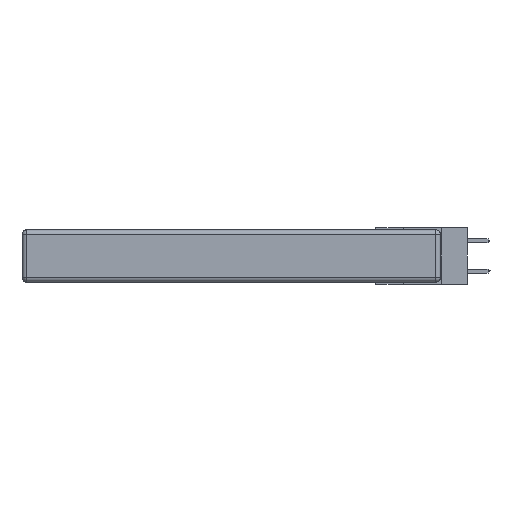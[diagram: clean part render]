
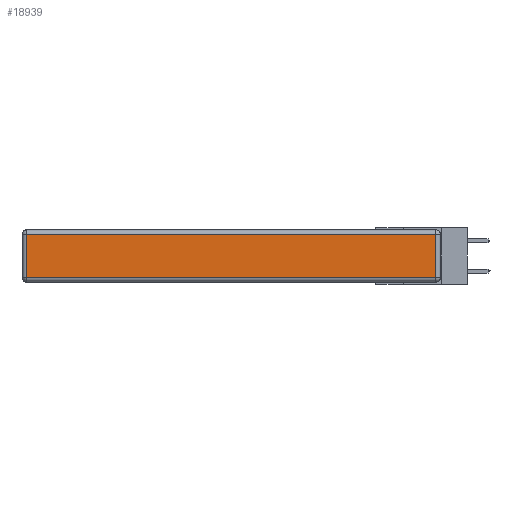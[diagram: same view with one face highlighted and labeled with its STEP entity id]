
A CAD part, left-side view. The second image highlights one B-rep face of the part: STEP entity #18939.
In plain terms, the highlighted planar face has unit normal (-1, 0, 0).
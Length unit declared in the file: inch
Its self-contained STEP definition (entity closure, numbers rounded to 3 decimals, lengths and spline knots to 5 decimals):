
#454 = ORIENTED_EDGE ( 'NONE', *, *, #20297, .T. ) ;
#1359 = ORIENTED_EDGE ( 'NONE', *, *, #7262, .T. ) ;
#4523 = AXIS2_PLACEMENT_3D ( 'NONE', #9905, #8316, #6566 ) ;
#4576 = CARTESIAN_POINT ( 'NONE',  ( 0., 2.72, -0.343 ) ) ;
#4876 = CARTESIAN_POINT ( 'NONE',  ( 0., 0.03, -0.313 ) ) ;
#4912 = FACE_OUTER_BOUND ( 'NONE', #19882, .T. ) ;
#5044 = CARTESIAN_POINT ( 'NONE',  ( 0., 0.03, -0.343 ) ) ;
#5182 = ORIENTED_EDGE ( 'NONE', *, *, #13146, .T. ) ;
#5830 = VECTOR ( 'NONE', #19994, 39.37008 ) ;
#6077 = DIRECTION ( 'NONE',  ( 0., 0., -1. ) ) ;
#6189 = CARTESIAN_POINT ( 'NONE',  ( 0., 0.03, -0.03 ) ) ;
#6566 = DIRECTION ( 'NONE',  ( 0., 0., 1. ) ) ;
#6700 = ORIENTED_EDGE ( 'NONE', *, *, #9604, .T. ) ;
#7262 = EDGE_CURVE ( 'NONE', #7684, #8375, #20512, .T. ) ;
#7684 = VERTEX_POINT ( 'NONE', #13353 ) ;
#8082 = VECTOR ( 'NONE', #8680, 39.37008 ) ;
#8316 = DIRECTION ( 'NONE',  ( -1., 0., 0. ) ) ;
#8375 = VERTEX_POINT ( 'NONE', #4876 ) ;
#8534 = LINE ( 'NONE', #16728, #5830 ) ;
#8680 = DIRECTION ( 'NONE',  ( 0., 0., 1. ) ) ;
#9604 = EDGE_CURVE ( 'NONE', #15154, #7684, #15481, .T. ) ;
#9905 = CARTESIAN_POINT ( 'NONE',  ( 0., 0., -0.343 ) ) ;
#10826 = VECTOR ( 'NONE', #6077, 39.37008 ) ;
#12897 = VECTOR ( 'NONE', #18544, 39.37008 ) ;
#13090 = VERTEX_POINT ( 'NONE', #6189 ) ;
#13146 = EDGE_CURVE ( 'NONE', #13090, #15154, #8534, .T. ) ;
#13353 = CARTESIAN_POINT ( 'NONE',  ( 0., 2.72, -0.313 ) ) ;
#15154 = VERTEX_POINT ( 'NONE', #19714 ) ;
#15481 = LINE ( 'NONE', #4576, #10826 ) ;
#15985 = CARTESIAN_POINT ( 'NONE',  ( 0., 0., -0.313 ) ) ;
#16728 = CARTESIAN_POINT ( 'NONE',  ( 0., 2.75, -0.03 ) ) ;
#17052 = PLANE ( 'NONE',  #4523 ) ;
#18544 = DIRECTION ( 'NONE',  ( 0., -1., 0. ) ) ;
#18939 = ADVANCED_FACE ( 'NONE', ( #4912 ), #17052, .T. ) ;
#19714 = CARTESIAN_POINT ( 'NONE',  ( 0., 2.72, -0.03 ) ) ;
#19882 = EDGE_LOOP ( 'NONE', ( #1359, #454, #5182, #6700 ) ) ;
#19994 = DIRECTION ( 'NONE',  ( 0., 1., 0. ) ) ;
#20297 = EDGE_CURVE ( 'NONE', #8375, #13090, #20377, .T. ) ;
#20377 = LINE ( 'NONE', #5044, #8082 ) ;
#20512 = LINE ( 'NONE', #15985, #12897 ) ;
